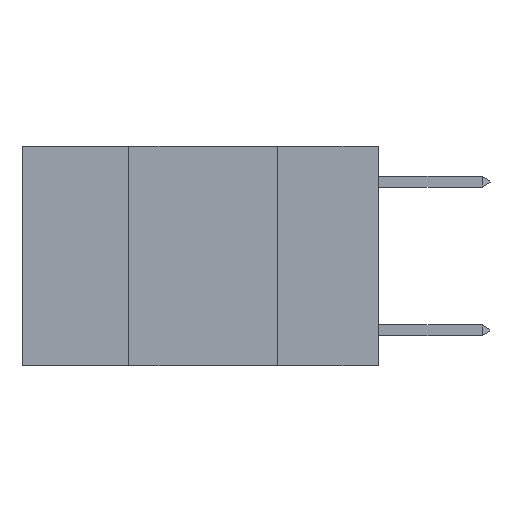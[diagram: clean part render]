
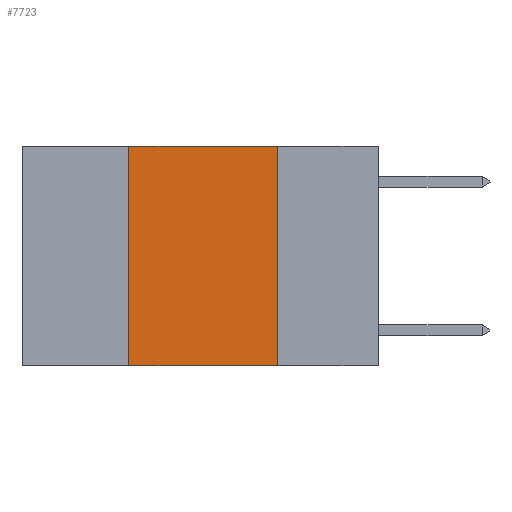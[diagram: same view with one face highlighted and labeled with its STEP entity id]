
A CAD part, left-side view. The second image highlights one B-rep face of the part: STEP entity #7723.
In plain terms, the highlighted planar face has unit normal (-1, 0, 0).
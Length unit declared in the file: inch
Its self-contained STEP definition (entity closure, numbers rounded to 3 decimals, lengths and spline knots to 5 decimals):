
#112 = LINE ( 'NONE', #1725, #18649 ) ;
#304 = CARTESIAN_POINT ( 'NONE',  ( 0., 0.6, 0. ) ) ;
#433 = VECTOR ( 'NONE', #2646, 39.37008 ) ;
#1316 = EDGE_LOOP ( 'NONE', ( #3619, #9346, #6311, #9582 ) ) ;
#1725 = CARTESIAN_POINT ( 'NONE',  ( 0., 0.6, 0. ) ) ;
#2646 = DIRECTION ( 'NONE',  ( 0., 0., -1. ) ) ;
#3123 = VERTEX_POINT ( 'NONE', #4336 ) ;
#3619 = ORIENTED_EDGE ( 'NONE', *, *, #22750, .F. ) ;
#4305 = VERTEX_POINT ( 'NONE', #11391 ) ;
#4336 = CARTESIAN_POINT ( 'NONE',  ( 0., 0.17, -0.37 ) ) ;
#4880 = LINE ( 'NONE', #8694, #10457 ) ;
#5413 = AXIS2_PLACEMENT_3D ( 'NONE', #304, #22391, #11527 ) ;
#6311 = ORIENTED_EDGE ( 'NONE', *, *, #11847, .F. ) ;
#7723 = ADVANCED_FACE ( 'NONE', ( #11489 ), #16988, .F. ) ;
#8694 = CARTESIAN_POINT ( 'NONE',  ( 0., 0.42, 0. ) ) ;
#9346 = ORIENTED_EDGE ( 'NONE', *, *, #23032, .F. ) ;
#9582 = ORIENTED_EDGE ( 'NONE', *, *, #20114, .T. ) ;
#10125 = VECTOR ( 'NONE', #14746, 39.37008 ) ;
#10326 = LINE ( 'NONE', #17508, #433 ) ;
#10457 = VECTOR ( 'NONE', #14270, 39.37008 ) ;
#11391 = CARTESIAN_POINT ( 'NONE',  ( 0., 0.42, 0. ) ) ;
#11489 = FACE_OUTER_BOUND ( 'NONE', #1316, .T. ) ;
#11527 = DIRECTION ( 'NONE',  ( 0., 0., -1. ) ) ;
#11847 = EDGE_CURVE ( 'NONE', #15902, #4305, #4880, .T. ) ;
#12879 = CARTESIAN_POINT ( 'NONE',  ( 0., 0.6, -0.37 ) ) ;
#13423 = CARTESIAN_POINT ( 'NONE',  ( 0., 0.42, -0.37 ) ) ;
#14270 = DIRECTION ( 'NONE',  ( 0., 0., 1. ) ) ;
#14746 = DIRECTION ( 'NONE',  ( 0., -1., 0. ) ) ;
#15728 = CARTESIAN_POINT ( 'NONE',  ( 0., 0.17, 0. ) ) ;
#15902 = VERTEX_POINT ( 'NONE', #13423 ) ;
#16567 = DIRECTION ( 'NONE',  ( 0., -1., 0. ) ) ;
#16988 = PLANE ( 'NONE',  #5413 ) ;
#17508 = CARTESIAN_POINT ( 'NONE',  ( 0., 0.17, 0. ) ) ;
#18649 = VECTOR ( 'NONE', #16567, 39.37008 ) ;
#19018 = VERTEX_POINT ( 'NONE', #15728 ) ;
#19878 = LINE ( 'NONE', #12879, #10125 ) ;
#20114 = EDGE_CURVE ( 'NONE', #15902, #3123, #19878, .T. ) ;
#22391 = DIRECTION ( 'NONE',  ( 1., 0., 0. ) ) ;
#22750 = EDGE_CURVE ( 'NONE', #19018, #3123, #10326, .T. ) ;
#23032 = EDGE_CURVE ( 'NONE', #4305, #19018, #112, .T. ) ;
